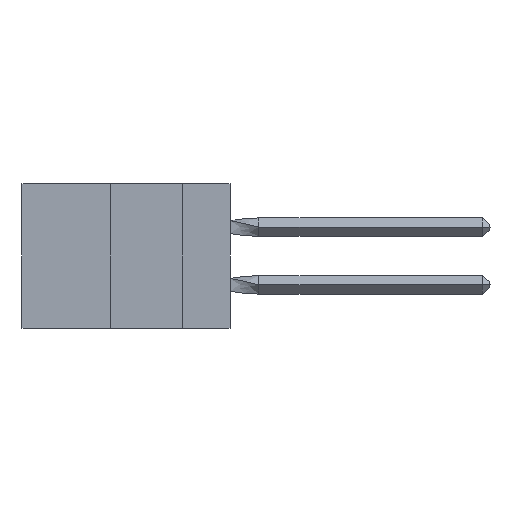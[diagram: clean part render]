
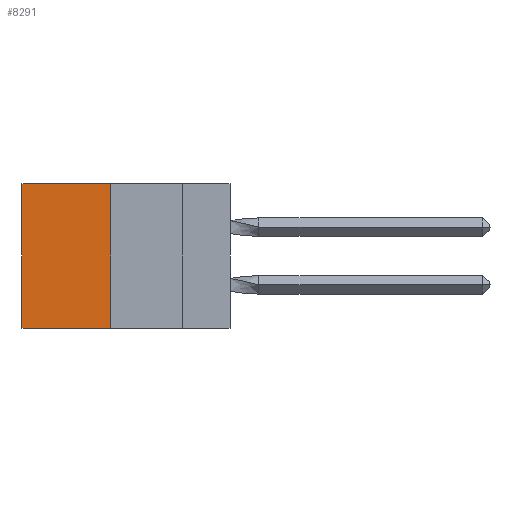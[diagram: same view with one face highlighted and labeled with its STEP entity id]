
A CAD part, left-side view. The second image highlights one B-rep face of the part: STEP entity #8291.
In plain terms, the highlighted planar face has unit normal (-1, 0, 0).
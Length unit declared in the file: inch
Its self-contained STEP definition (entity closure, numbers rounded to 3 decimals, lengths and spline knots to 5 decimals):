
#182 = CARTESIAN_POINT ( 'NONE',  ( 0.305, 0.413, -0.5 ) ) ;
#379 = EDGE_CURVE ( 'NONE', #12183, #9850, #12981, .T. ) ;
#1155 = CARTESIAN_POINT ( 'NONE',  ( 0.305, 0.413, 0. ) ) ;
#1218 = VERTEX_POINT ( 'NONE', #1831 ) ;
#1231 = CARTESIAN_POINT ( 'NONE',  ( 0.305, 0.413, 0. ) ) ;
#1273 = LINE ( 'NONE', #15322, #8674 ) ;
#1831 = CARTESIAN_POINT ( 'NONE',  ( 0.305, 0.72, -0.5 ) ) ;
#2411 = DIRECTION ( 'NONE',  ( 0., 1., 0. ) ) ;
#2977 = ORIENTED_EDGE ( 'NONE', *, *, #15590, .F. ) ;
#3700 = EDGE_CURVE ( 'NONE', #10643, #1218, #1273, .T. ) ;
#5269 = DIRECTION ( 'NONE',  ( 0., 0., -1. ) ) ;
#6160 = ORIENTED_EDGE ( 'NONE', *, *, #10964, .T. ) ;
#6536 = EDGE_LOOP ( 'NONE', ( #9515, #2977, #7712, #6160 ) ) ;
#6789 = CARTESIAN_POINT ( 'NONE',  ( 0.305, 0.413, -0.5 ) ) ;
#7142 = VECTOR ( 'NONE', #10906, 39.37008 ) ;
#7324 = LINE ( 'NONE', #14248, #7142 ) ;
#7712 = ORIENTED_EDGE ( 'NONE', *, *, #379, .F. ) ;
#8291 = ADVANCED_FACE ( 'NONE', ( #10873 ), #14177, .F. ) ;
#8674 = VECTOR ( 'NONE', #5269, 39.37008 ) ;
#9346 = DIRECTION ( 'NONE',  ( 0., 0., -1. ) ) ;
#9515 = ORIENTED_EDGE ( 'NONE', *, *, #3700, .T. ) ;
#9850 = VERTEX_POINT ( 'NONE', #182 ) ;
#10611 = VECTOR ( 'NONE', #2411, 39.37008 ) ;
#10643 = VERTEX_POINT ( 'NONE', #15394 ) ;
#10873 = FACE_OUTER_BOUND ( 'NONE', #6536, .T. ) ;
#10906 = DIRECTION ( 'NONE',  ( 0., 1., 0. ) ) ;
#10964 = EDGE_CURVE ( 'NONE', #12183, #10643, #15713, .T. ) ;
#11880 = CARTESIAN_POINT ( 'NONE',  ( 0.305, 0.413, -0.5 ) ) ;
#12183 = VERTEX_POINT ( 'NONE', #1231 ) ;
#12981 = LINE ( 'NONE', #6789, #15309 ) ;
#14177 = PLANE ( 'NONE',  #14935 ) ;
#14248 = CARTESIAN_POINT ( 'NONE',  ( 0.305, 0.413, -0.5 ) ) ;
#14393 = DIRECTION ( 'NONE',  ( 1., 0., 0. ) ) ;
#14935 = AXIS2_PLACEMENT_3D ( 'NONE', #11880, #14393, #15378 ) ;
#15309 = VECTOR ( 'NONE', #9346, 39.37008 ) ;
#15322 = CARTESIAN_POINT ( 'NONE',  ( 0.305, 0.72, -0.5 ) ) ;
#15378 = DIRECTION ( 'NONE',  ( 0., 0., -1. ) ) ;
#15394 = CARTESIAN_POINT ( 'NONE',  ( 0.305, 0.72, 0. ) ) ;
#15590 = EDGE_CURVE ( 'NONE', #9850, #1218, #7324, .T. ) ;
#15713 = LINE ( 'NONE', #1155, #10611 ) ;
